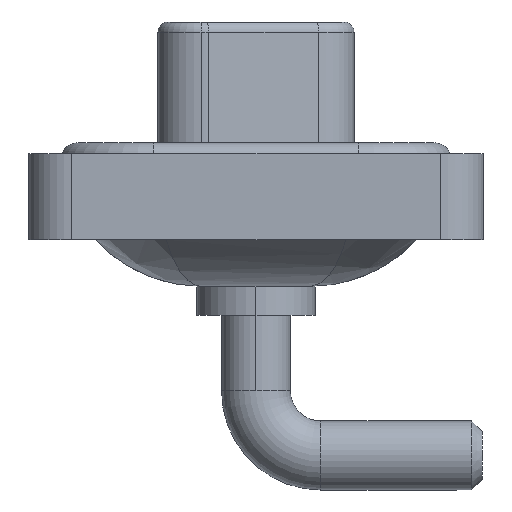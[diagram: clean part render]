
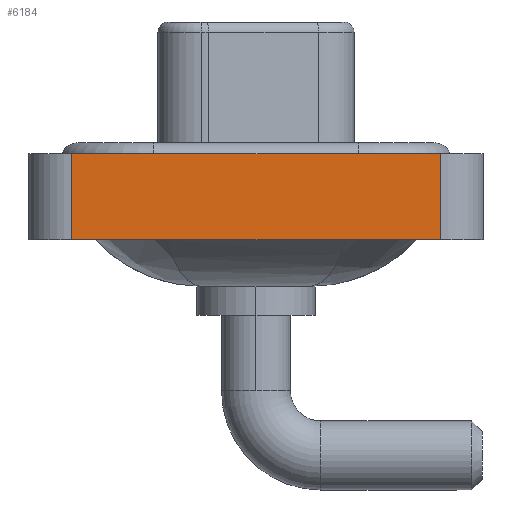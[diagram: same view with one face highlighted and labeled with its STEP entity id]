
A CAD part, left-side view. The second image highlights one B-rep face of the part: STEP entity #6184.
In plain terms, the highlighted planar face has unit normal (-1, 0, 0).
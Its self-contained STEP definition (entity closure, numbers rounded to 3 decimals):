
#109 = VECTOR ( 'NONE', #5888, 1000. ) ;
#452 = EDGE_LOOP ( 'NONE', ( #4675, #16696, #15287, #14404 ) ) ;
#533 = EDGE_CURVE ( 'NONE', #10725, #16132, #8673, .T. ) ;
#1191 = VECTOR ( 'NONE', #4326, 1000. ) ;
#1200 = CARTESIAN_POINT ( 'NONE',  ( -7.25, -8.55, -3.6 ) ) ;
#2011 = CARTESIAN_POINT ( 'NONE',  ( -7.25, -8.55, 0.4 ) ) ;
#2901 = LINE ( 'NONE', #11305, #109 ) ;
#2995 = AXIS2_PLACEMENT_3D ( 'NONE', #1200, #8267, #8179 ) ;
#4020 = CARTESIAN_POINT ( 'NONE',  ( -7.25, -8.55, -3.6 ) ) ;
#4326 = DIRECTION ( 'NONE',  ( 0., 0., 1. ) ) ;
#4675 = ORIENTED_EDGE ( 'NONE', *, *, #15871, .T. ) ;
#5102 = VECTOR ( 'NONE', #12651, 1000. ) ;
#5244 = CARTESIAN_POINT ( 'NONE',  ( -7.25, 8.55, 0.4 ) ) ;
#5808 = LINE ( 'NONE', #7430, #13488 ) ;
#5888 = DIRECTION ( 'NONE',  ( 0., -1., 0. ) ) ;
#6184 = ADVANCED_FACE ( 'NONE', ( #12228 ), #9710, .T. ) ;
#7430 = CARTESIAN_POINT ( 'NONE',  ( -7.25, 8.55, -3.6 ) ) ;
#8179 = DIRECTION ( 'NONE',  ( 0., 0., 1. ) ) ;
#8267 = DIRECTION ( 'NONE',  ( -1., 0., 0. ) ) ;
#8673 = LINE ( 'NONE', #11199, #5102 ) ;
#9710 = PLANE ( 'NONE',  #2995 ) ;
#9790 = DIRECTION ( 'NONE',  ( 0., 0., 1. ) ) ;
#10725 = VERTEX_POINT ( 'NONE', #11278 ) ;
#11199 = CARTESIAN_POINT ( 'NONE',  ( -7.25, -8.55, -3.6 ) ) ;
#11278 = CARTESIAN_POINT ( 'NONE',  ( -7.25, 8.55, -3.6 ) ) ;
#11305 = CARTESIAN_POINT ( 'NONE',  ( -7.25, -8.55, 0.4 ) ) ;
#11665 = VERTEX_POINT ( 'NONE', #2011 ) ;
#12228 = FACE_OUTER_BOUND ( 'NONE', #452, .T. ) ;
#12356 = EDGE_CURVE ( 'NONE', #10725, #13599, #5808, .T. ) ;
#12545 = CARTESIAN_POINT ( 'NONE',  ( -7.25, -8.55, -3.6 ) ) ;
#12651 = DIRECTION ( 'NONE',  ( 0., -1., 0. ) ) ;
#13488 = VECTOR ( 'NONE', #9790, 1000. ) ;
#13599 = VERTEX_POINT ( 'NONE', #5244 ) ;
#14081 = LINE ( 'NONE', #12545, #1191 ) ;
#14404 = ORIENTED_EDGE ( 'NONE', *, *, #533, .T. ) ;
#15287 = ORIENTED_EDGE ( 'NONE', *, *, #12356, .F. ) ;
#15871 = EDGE_CURVE ( 'NONE', #16132, #11665, #14081, .T. ) ;
#16132 = VERTEX_POINT ( 'NONE', #4020 ) ;
#16696 = ORIENTED_EDGE ( 'NONE', *, *, #17267, .F. ) ;
#17267 = EDGE_CURVE ( 'NONE', #13599, #11665, #2901, .T. ) ;
